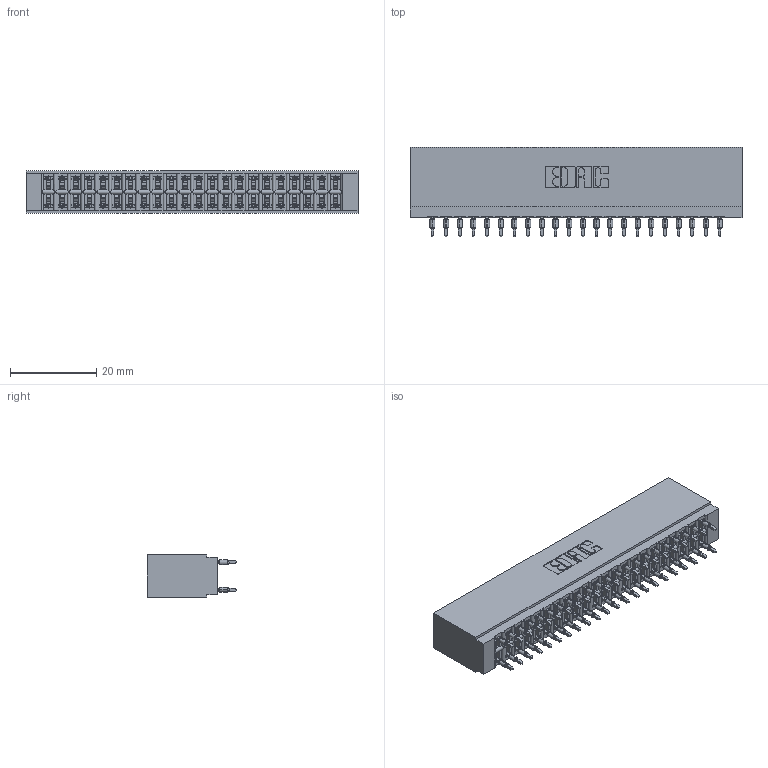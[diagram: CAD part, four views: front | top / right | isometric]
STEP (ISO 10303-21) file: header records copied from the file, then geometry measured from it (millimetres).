
FILE_DESCRIPTION (( 'STEP AP203' ), '1' );
FILE_NAME ('746-044-560-201.STEP', '2026-02-27T15:00:21', ( '' ), ( '' ), 'SwSTEP 2.0', 'SolidWorks 2023', '' );
FILE_SCHEMA (( 'CONFIG_CONTROL_DESIGN' ));
Length unit declared in the file: millimetre
Products named in the file (3): 746-044-560-201; 746-292-001_560; 746 Part_.515 Slot Depth - 01
Assembly tree (45 placements, depth 2):
  746-044-560-201
    746 Part_.515 Slot Depth - 01
    746-292-001_560  x44
Bounding box: 77.09 x 20.82 x 9.91 mm (x, y, z)
Volume: 8544.3 mm3; surface area: 14036.4 mm2
Topology: 45 solids, 45 shells, 4255 faces, 11835 edges, 7589 vertices
Faces by surface type: plane 2123, cylinder 988, bspline 880, torus 264
Entity records: 36960 total; most frequent: CARTESIAN_POINT 7519, ORIENTED_EDGE 6298, DIRECTION 5299, EDGE_CURVE 3149, LINE 2737, VECTOR 2737, VERTEX_POINT 2085, AXIS2_PLACEMENT_3D 1281
